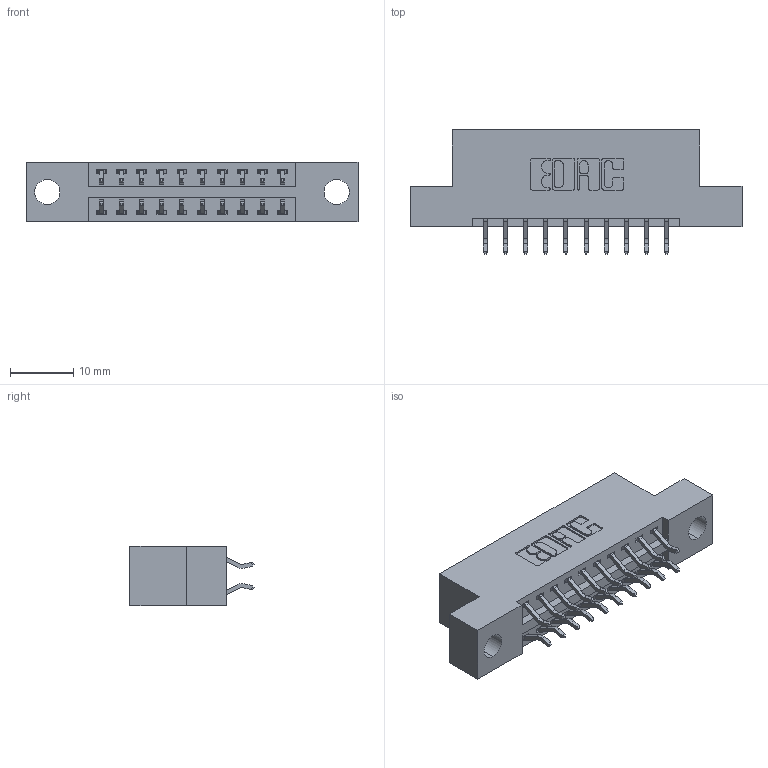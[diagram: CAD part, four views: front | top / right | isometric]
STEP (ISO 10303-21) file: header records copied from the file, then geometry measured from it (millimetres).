
FILE_DESCRIPTION (( 'STEP AP203' ), '1' );
FILE_NAME ('346-020-556-204.STEP', '2022-05-18T19:46:06', ( '' ), ( '' ), 'SwSTEP 2.0', 'SolidWorks 2020', '' );
FILE_SCHEMA (( 'CONFIG_CONTROL_DESIGN' ));
Length unit declared in the file: inch
Products named in the file (3): 346 Part_Flush Mounting Lugs - 0.156 Dia-TH; 346-020-556-204; 345-292-001_556 Tail
Assembly tree (21 placements, depth 2):
  346-020-556-204
    346 Part_Flush Mounting Lugs - 0.156 Dia-TH
    345-292-001_556 Tail  x20
Bounding box: 52.32 x 19.57 x 9.4 mm (x, y, z)
Volume: 4747 mm3; surface area: 5851.4 mm2
Topology: 21 solids, 21 shells, 1296 faces, 3825 edges, 2522 vertices
Faces by surface type: plane 870, cylinder 426
Entity records: 11473 total; most frequent: CARTESIAN_POINT 1954, ORIENTED_EDGE 1874, DIRECTION 1761, EDGE_CURVE 937, LINE 757, VECTOR 757, VERTEX_POINT 622, AXIS2_PLACEMENT_3D 502
